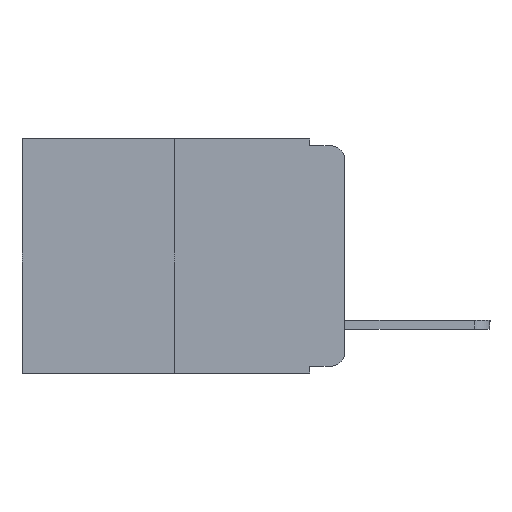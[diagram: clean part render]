
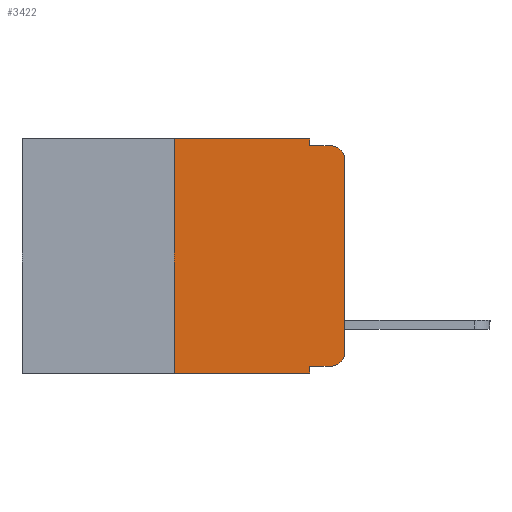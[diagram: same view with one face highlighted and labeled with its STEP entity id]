
A CAD part, left-side view. The second image highlights one B-rep face of the part: STEP entity #3422.
In plain terms, the highlighted planar face has unit normal (-1, 0, 0).
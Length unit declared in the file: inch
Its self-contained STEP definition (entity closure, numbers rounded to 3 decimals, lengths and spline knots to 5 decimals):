
#179 = DIRECTION ( 'NONE',  ( 0., 0., -1. ) ) ;
#448 = DIRECTION ( 'NONE',  ( 0., -1., 0. ) ) ;
#567 = VECTOR ( 'NONE', #3429, 39.37008 ) ;
#750 = DIRECTION ( 'NONE',  ( 0., 0., -1. ) ) ;
#882 = FACE_OUTER_BOUND ( 'NONE', #17958, .T. ) ;
#894 = ORIENTED_EDGE ( 'NONE', *, *, #14302, .T. ) ;
#984 = ORIENTED_EDGE ( 'NONE', *, *, #3563, .F. ) ;
#1413 = DIRECTION ( 'NONE',  ( 1., 0., 0. ) ) ;
#1624 = AXIS2_PLACEMENT_3D ( 'NONE', #8102, #20586, #179 ) ;
#1681 = EDGE_CURVE ( 'NONE', #2041, #7699, #12139, .T. ) ;
#1819 = EDGE_CURVE ( 'NONE', #17723, #7699, #18986, .T. ) ;
#1942 = EDGE_CURVE ( 'NONE', #17723, #18632, #6864, .T. ) ;
#2041 = VERTEX_POINT ( 'NONE', #14180 ) ;
#2420 = DIRECTION ( 'NONE',  ( 0., 0., 1. ) ) ;
#2996 = ORIENTED_EDGE ( 'NONE', *, *, #6158, .T. ) ;
#3025 = ORIENTED_EDGE ( 'NONE', *, *, #1681, .F. ) ;
#3073 = EDGE_CURVE ( 'NONE', #7502, #6052, #10573, .T. ) ;
#3422 = ADVANCED_FACE ( 'NONE', ( #882 ), #17222, .F. ) ;
#3429 = DIRECTION ( 'NONE',  ( 0., -1., 0. ) ) ;
#3563 = EDGE_CURVE ( 'NONE', #18632, #14061, #6332, .T. ) ;
#3748 = ORIENTED_EDGE ( 'NONE', *, *, #4836, .F. ) ;
#3754 = DIRECTION ( 'NONE',  ( 0., -1., 0. ) ) ;
#4409 = VECTOR ( 'NONE', #750, 39.37008 ) ;
#4760 = ORIENTED_EDGE ( 'NONE', *, *, #1942, .F. ) ;
#4836 = EDGE_CURVE ( 'NONE', #14061, #15981, #18132, .T. ) ;
#5239 = CARTESIAN_POINT ( 'NONE',  ( 0., 0.25, 0. ) ) ;
#5484 = CARTESIAN_POINT ( 'NONE',  ( 0., 0.25, -0.343 ) ) ;
#5604 = CARTESIAN_POINT ( 'NONE',  ( 0., 0.02, -0.313 ) ) ;
#6052 = VERTEX_POINT ( 'NONE', #11821 ) ;
#6158 = EDGE_CURVE ( 'NONE', #18638, #8694, #12985, .T. ) ;
#6220 = CARTESIAN_POINT ( 'NONE',  ( 0., 0.473, 0. ) ) ;
#6332 = LINE ( 'NONE', #7035, #9810 ) ;
#6692 = EDGE_CURVE ( 'NONE', #15981, #6052, #9272, .T. ) ;
#6800 = EDGE_CURVE ( 'NONE', #2041, #18638, #19321, .T. ) ;
#6864 = LINE ( 'NONE', #10162, #10545 ) ;
#6892 = CARTESIAN_POINT ( 'NONE',  ( 0., 0.051, -0.333 ) ) ;
#7035 = CARTESIAN_POINT ( 'NONE',  ( 0., 0.473, 0. ) ) ;
#7051 = VECTOR ( 'NONE', #11557, 39.37008 ) ;
#7502 = VERTEX_POINT ( 'NONE', #20123 ) ;
#7684 = CARTESIAN_POINT ( 'NONE',  ( 0., 0.473, -0.343 ) ) ;
#7699 = VERTEX_POINT ( 'NONE', #19179 ) ;
#7805 = ORIENTED_EDGE ( 'NONE', *, *, #6800, .T. ) ;
#8102 = CARTESIAN_POINT ( 'NONE',  ( 0., 0.02, -0.03 ) ) ;
#8674 = CARTESIAN_POINT ( 'NONE',  ( 0., 0., 0. ) ) ;
#8694 = VERTEX_POINT ( 'NONE', #10993 ) ;
#9017 = VECTOR ( 'NONE', #3754, 39.37008 ) ;
#9272 = LINE ( 'NONE', #15617, #9017 ) ;
#9810 = VECTOR ( 'NONE', #448, 39.37008 ) ;
#9858 = CARTESIAN_POINT ( 'NONE',  ( 0., 0.051, 0. ) ) ;
#10162 = CARTESIAN_POINT ( 'NONE',  ( 0., 0.25, 0. ) ) ;
#10333 = LINE ( 'NONE', #8674, #14879 ) ;
#10545 = VECTOR ( 'NONE', #11419, 39.37008 ) ;
#10573 = CIRCLE ( 'NONE', #1624, 0.02 ) ;
#10993 = CARTESIAN_POINT ( 'NONE',  ( 0., 0., -0.313 ) ) ;
#11419 = DIRECTION ( 'NONE',  ( 0., 0., 1. ) ) ;
#11545 = VECTOR ( 'NONE', #13923, 39.37008 ) ;
#11557 = DIRECTION ( 'NONE',  ( 0., -1., 0. ) ) ;
#11567 = CARTESIAN_POINT ( 'NONE',  ( 0., 0.02, -0.333 ) ) ;
#11821 = CARTESIAN_POINT ( 'NONE',  ( 0., 0.02, -0.01 ) ) ;
#11922 = DIRECTION ( 'NONE',  ( 0., 0., -1. ) ) ;
#12139 = LINE ( 'NONE', #16928, #11545 ) ;
#12985 = CIRCLE ( 'NONE', #19600, 0.02 ) ;
#13685 = DIRECTION ( 'NONE',  ( -1., 0., 0. ) ) ;
#13923 = DIRECTION ( 'NONE',  ( 0., 0., -1. ) ) ;
#14061 = VERTEX_POINT ( 'NONE', #18968 ) ;
#14180 = CARTESIAN_POINT ( 'NONE',  ( 0., 0.051, -0.333 ) ) ;
#14302 = EDGE_CURVE ( 'NONE', #8694, #7502, #10333, .T. ) ;
#14879 = VECTOR ( 'NONE', #2420, 39.37008 ) ;
#15617 = CARTESIAN_POINT ( 'NONE',  ( 0., 0.051, -0.01 ) ) ;
#15981 = VERTEX_POINT ( 'NONE', #16064 ) ;
#16064 = CARTESIAN_POINT ( 'NONE',  ( 0., 0.051, -0.01 ) ) ;
#16653 = ORIENTED_EDGE ( 'NONE', *, *, #6692, .F. ) ;
#16928 = CARTESIAN_POINT ( 'NONE',  ( 0., 0.051, 0. ) ) ;
#17222 = PLANE ( 'NONE',  #19555 ) ;
#17723 = VERTEX_POINT ( 'NONE', #5484 ) ;
#17958 = EDGE_LOOP ( 'NONE', ( #894, #19022, #16653, #3748, #984, #4760, #18344, #3025, #7805, #2996 ) ) ;
#18132 = LINE ( 'NONE', #9858, #4409 ) ;
#18344 = ORIENTED_EDGE ( 'NONE', *, *, #1819, .T. ) ;
#18632 = VERTEX_POINT ( 'NONE', #5239 ) ;
#18638 = VERTEX_POINT ( 'NONE', #11567 ) ;
#18968 = CARTESIAN_POINT ( 'NONE',  ( 0., 0.051, 0. ) ) ;
#18986 = LINE ( 'NONE', #7684, #567 ) ;
#19022 = ORIENTED_EDGE ( 'NONE', *, *, #3073, .T. ) ;
#19179 = CARTESIAN_POINT ( 'NONE',  ( 0., 0.051, -0.343 ) ) ;
#19321 = LINE ( 'NONE', #6892, #7051 ) ;
#19555 = AXIS2_PLACEMENT_3D ( 'NONE', #6220, #1413, #20443 ) ;
#19600 = AXIS2_PLACEMENT_3D ( 'NONE', #5604, #13685, #11922 ) ;
#20123 = CARTESIAN_POINT ( 'NONE',  ( 0., 0., -0.03 ) ) ;
#20443 = DIRECTION ( 'NONE',  ( 0., 0., -1. ) ) ;
#20586 = DIRECTION ( 'NONE',  ( -1., 0., 0. ) ) ;
